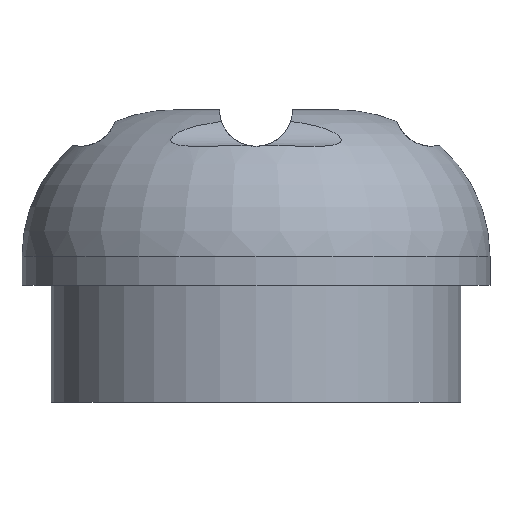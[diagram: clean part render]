
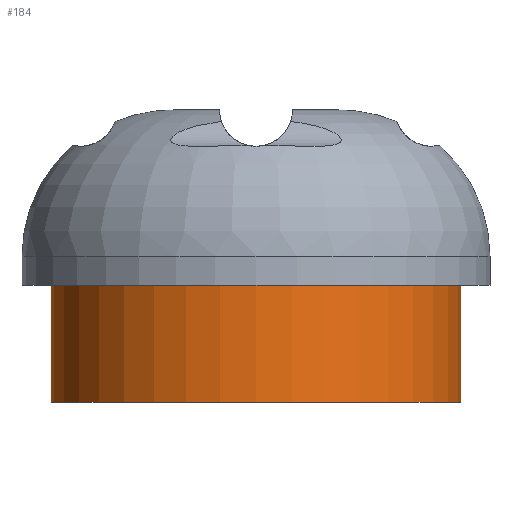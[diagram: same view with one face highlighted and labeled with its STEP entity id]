
A CAD part, front view. The second image highlights one B-rep face of the part: STEP entity #184.
In plain terms, the highlighted cylindrical face has radius 3.5 mm (diameter 7 mm), a partial arc.
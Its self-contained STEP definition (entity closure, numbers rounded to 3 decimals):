
#21 = DIRECTION ( 'NONE',  ( 0., 0., -1. ) ) ;
#61 = CARTESIAN_POINT ( 'NONE',  ( 0., 0., 0. ) ) ;
#130 = DIRECTION ( 'NONE',  ( 1., 0., 0. ) ) ;
#184 = ADVANCED_FACE ( 'NONE', ( #798 ), #787, .T. ) ;
#233 = CARTESIAN_POINT ( 'NONE',  ( 0., 0., 2. ) ) ;
#238 = CARTESIAN_POINT ( 'NONE',  ( -3.5, 0., 2. ) ) ;
#288 = DIRECTION ( 'NONE',  ( 1., 0., 0. ) ) ;
#330 = CARTESIAN_POINT ( 'NONE',  ( 3.5, 0., 2. ) ) ;
#376 = DIRECTION ( 'NONE',  ( 0., 0., -1. ) ) ;
#489 = DIRECTION ( 'NONE',  ( -1., 0., 0. ) ) ;
#535 = DIRECTION ( 'NONE',  ( 0., 0., 1. ) ) ;
#542 = AXIS2_PLACEMENT_3D ( 'NONE', #61, #535, #130 ) ;
#597 = EDGE_CURVE ( 'NONE', #1124, #991, #692, .T. ) ;
#605 = CARTESIAN_POINT ( 'NONE',  ( -3.5, 0., 0. ) ) ;
#624 = EDGE_CURVE ( 'NONE', #1013, #991, #680, .T. ) ;
#626 = VECTOR ( 'NONE', #856, 1000. ) ;
#632 = LINE ( 'NONE', #998, #626 ) ;
#657 = CIRCLE ( 'NONE', #1119, 3.5 ) ;
#680 = CIRCLE ( 'NONE', #542, 3.5 ) ;
#691 = VECTOR ( 'NONE', #376, 1000. ) ;
#692 = LINE ( 'NONE', #969, #691 ) ;
#773 = DIRECTION ( 'NONE',  ( 0., 0., 1. ) ) ;
#787 = CYLINDRICAL_SURFACE ( 'NONE', #982, 3.5 ) ;
#798 = FACE_OUTER_BOUND ( 'NONE', #1141, .T. ) ;
#815 = CARTESIAN_POINT ( 'NONE',  ( 3.5, 0., 0. ) ) ;
#840 = EDGE_CURVE ( 'NONE', #912, #1124, #657, .T. ) ;
#856 = DIRECTION ( 'NONE',  ( 0., 0., -1. ) ) ;
#870 = ORIENTED_EDGE ( 'NONE', *, *, #597, .F. ) ;
#878 = CARTESIAN_POINT ( 'NONE',  ( 0., 0., 2. ) ) ;
#898 = ORIENTED_EDGE ( 'NONE', *, *, #624, .T. ) ;
#912 = VERTEX_POINT ( 'NONE', #238 ) ;
#969 = CARTESIAN_POINT ( 'NONE',  ( 3.5, 0., 2. ) ) ;
#982 = AXIS2_PLACEMENT_3D ( 'NONE', #878, #21, #489 ) ;
#985 = ORIENTED_EDGE ( 'NONE', *, *, #1028, .T. ) ;
#991 = VERTEX_POINT ( 'NONE', #815 ) ;
#998 = CARTESIAN_POINT ( 'NONE',  ( -3.5, 0., 2. ) ) ;
#1013 = VERTEX_POINT ( 'NONE', #605 ) ;
#1028 = EDGE_CURVE ( 'NONE', #912, #1013, #632, .T. ) ;
#1089 = ORIENTED_EDGE ( 'NONE', *, *, #840, .F. ) ;
#1119 = AXIS2_PLACEMENT_3D ( 'NONE', #233, #773, #288 ) ;
#1124 = VERTEX_POINT ( 'NONE', #330 ) ;
#1141 = EDGE_LOOP ( 'NONE', ( #870, #1089, #985, #898 ) ) ;
